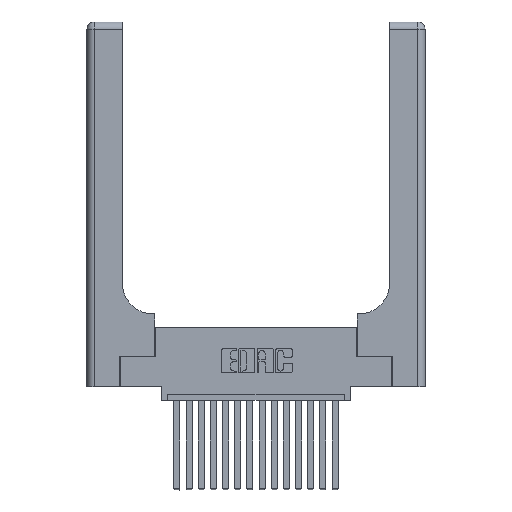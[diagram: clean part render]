
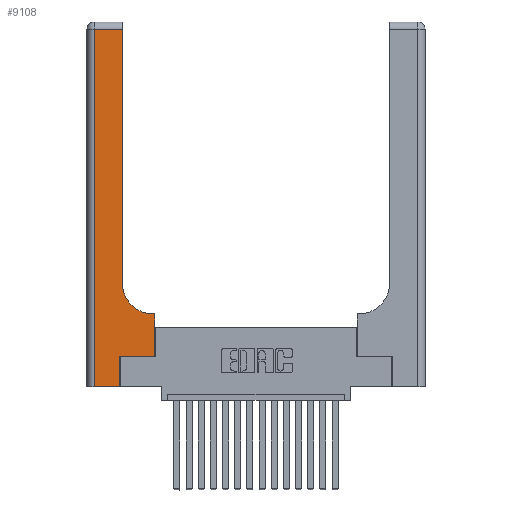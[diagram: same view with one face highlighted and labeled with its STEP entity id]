
A CAD part, top view. The second image highlights one B-rep face of the part: STEP entity #9108.
In plain terms, the highlighted planar face has unit normal (0, 0, 1).
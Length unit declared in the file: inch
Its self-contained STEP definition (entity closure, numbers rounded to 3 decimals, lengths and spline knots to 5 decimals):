
#108 = DIRECTION ( 'NONE',  ( 0., 0., -1. ) ) ;
#200 = DIRECTION ( 'NONE',  ( 0., -1., 0. ) ) ;
#417 = VECTOR ( 'NONE', #13288, 39.37008 ) ;
#592 = VECTOR ( 'NONE', #13034, 39.37008 ) ;
#596 = AXIS2_PLACEMENT_3D ( 'NONE', #1285, #13257, #5151 ) ;
#868 = VERTEX_POINT ( 'NONE', #9529 ) ;
#1285 = CARTESIAN_POINT ( 'NONE',  ( 0., 3., 0.37 ) ) ;
#1529 = DIRECTION ( 'NONE',  ( 1., 0., 0. ) ) ;
#1551 = CARTESIAN_POINT ( 'NONE',  ( 0.269, 0.25, 0.37 ) ) ;
#1599 = CARTESIAN_POINT ( 'NONE',  ( 0.269, 0.25, 0.37 ) ) ;
#1839 = DIRECTION ( 'NONE',  ( 0., 1., 0. ) ) ;
#1904 = ORIENTED_EDGE ( 'NONE', *, *, #16766, .T. ) ;
#2016 = EDGE_CURVE ( 'NONE', #11060, #5729, #15123, .T. ) ;
#2225 = VECTOR ( 'NONE', #15488, 39.37008 ) ;
#2803 = CARTESIAN_POINT ( 'NONE',  ( 0., 2.94, 0.37 ) ) ;
#2957 = VERTEX_POINT ( 'NONE', #4611 ) ;
#3359 = LINE ( 'NONE', #16279, #4289 ) ;
#3523 = VERTEX_POINT ( 'NONE', #14017 ) ;
#3643 = EDGE_CURVE ( 'NONE', #3523, #8258, #3359, .T. ) ;
#4289 = VECTOR ( 'NONE', #19315, 39.37008 ) ;
#4581 = LINE ( 'NONE', #1599, #16082 ) ;
#4611 = CARTESIAN_POINT ( 'NONE',  ( 0.269, 0., 0.37 ) ) ;
#4952 = CARTESIAN_POINT ( 'NONE',  ( 0., 0., 0.37 ) ) ;
#5151 = DIRECTION ( 'NONE',  ( -1., 0., 0. ) ) ;
#5155 = ORIENTED_EDGE ( 'NONE', *, *, #18055, .T. ) ;
#5550 = CARTESIAN_POINT ( 'NONE',  ( 0.06, 0., 0.37 ) ) ;
#5729 = VERTEX_POINT ( 'NONE', #11449 ) ;
#6021 = CARTESIAN_POINT ( 'NONE',  ( 0.06, 3., 0.37 ) ) ;
#6549 = DIRECTION ( 'NONE',  ( 1., 0., 0. ) ) ;
#6673 = LINE ( 'NONE', #4952, #19106 ) ;
#7007 = EDGE_CURVE ( 'NONE', #8258, #868, #15185, .T. ) ;
#8133 = LINE ( 'NONE', #6021, #18205 ) ;
#8258 = VERTEX_POINT ( 'NONE', #18296 ) ;
#8805 = ORIENTED_EDGE ( 'NONE', *, *, #10904, .T. ) ;
#8991 = ORIENTED_EDGE ( 'NONE', *, *, #15183, .T. ) ;
#9090 = EDGE_LOOP ( 'NONE', ( #8991, #16227, #5155, #15084, #12745, #8805, #17786, #16413, #1904 ) ) ;
#9108 = ADVANCED_FACE ( 'NONE', ( #15605 ), #11768, .F. ) ;
#9386 = CARTESIAN_POINT ( 'NONE',  ( 0.2915, 0.6, 0.37 ) ) ;
#9529 = CARTESIAN_POINT ( 'NONE',  ( 0.5415, 0.6, 0.37 ) ) ;
#10904 = EDGE_CURVE ( 'NONE', #17407, #3523, #4581, .T. ) ;
#11060 = VERTEX_POINT ( 'NONE', #17011 ) ;
#11449 = CARTESIAN_POINT ( 'NONE',  ( 0.06, 2.94, 0.37 ) ) ;
#11768 = PLANE ( 'NONE',  #596 ) ;
#12495 = VECTOR ( 'NONE', #1839, 39.37008 ) ;
#12745 = ORIENTED_EDGE ( 'NONE', *, *, #19031, .T. ) ;
#13034 = DIRECTION ( 'NONE',  ( 0., 1., 0. ) ) ;
#13257 = DIRECTION ( 'NONE',  ( 0., 0., -1. ) ) ;
#13288 = DIRECTION ( 'NONE',  ( -1., 0., 0. ) ) ;
#13362 = VERTEX_POINT ( 'NONE', #18334 ) ;
#14017 = CARTESIAN_POINT ( 'NONE',  ( 0.5585, 0.25, 0.37 ) ) ;
#14643 = LINE ( 'NONE', #14790, #592 ) ;
#14790 = CARTESIAN_POINT ( 'NONE',  ( 0.269, 0., 0.37 ) ) ;
#15035 = CARTESIAN_POINT ( 'NONE',  ( 0.5415, 0.85, 0.37 ) ) ;
#15084 = ORIENTED_EDGE ( 'NONE', *, *, #18770, .T. ) ;
#15123 = LINE ( 'NONE', #2803, #2225 ) ;
#15183 = EDGE_CURVE ( 'NONE', #13362, #11060, #19039, .T. ) ;
#15185 = LINE ( 'NONE', #9386, #417 ) ;
#15192 = CARTESIAN_POINT ( 'NONE',  ( 0.2915, 3., 0.37 ) ) ;
#15488 = DIRECTION ( 'NONE',  ( -1., 0., 0. ) ) ;
#15605 = FACE_OUTER_BOUND ( 'NONE', #9090, .T. ) ;
#16082 = VECTOR ( 'NONE', #1529, 39.37008 ) ;
#16227 = ORIENTED_EDGE ( 'NONE', *, *, #2016, .T. ) ;
#16279 = CARTESIAN_POINT ( 'NONE',  ( 0.5585, 0.25, 0.37 ) ) ;
#16380 = CIRCLE ( 'NONE', #16672, 0.25 ) ;
#16413 = ORIENTED_EDGE ( 'NONE', *, *, #7007, .T. ) ;
#16672 = AXIS2_PLACEMENT_3D ( 'NONE', #15035, #108, #17798 ) ;
#16766 = EDGE_CURVE ( 'NONE', #868, #13362, #16380, .T. ) ;
#17011 = CARTESIAN_POINT ( 'NONE',  ( 0.2915, 2.94, 0.37 ) ) ;
#17407 = VERTEX_POINT ( 'NONE', #1551 ) ;
#17786 = ORIENTED_EDGE ( 'NONE', *, *, #3643, .T. ) ;
#17798 = DIRECTION ( 'NONE',  ( 1., 0., 0. ) ) ;
#17813 = VERTEX_POINT ( 'NONE', #5550 ) ;
#18055 = EDGE_CURVE ( 'NONE', #5729, #17813, #8133, .T. ) ;
#18205 = VECTOR ( 'NONE', #200, 39.37008 ) ;
#18296 = CARTESIAN_POINT ( 'NONE',  ( 0.5585, 0.6, 0.37 ) ) ;
#18334 = CARTESIAN_POINT ( 'NONE',  ( 0.2915, 0.85, 0.37 ) ) ;
#18770 = EDGE_CURVE ( 'NONE', #17813, #2957, #6673, .T. ) ;
#19031 = EDGE_CURVE ( 'NONE', #2957, #17407, #14643, .T. ) ;
#19039 = LINE ( 'NONE', #15192, #12495 ) ;
#19106 = VECTOR ( 'NONE', #6549, 39.37008 ) ;
#19315 = DIRECTION ( 'NONE',  ( 0., 1., 0. ) ) ;
